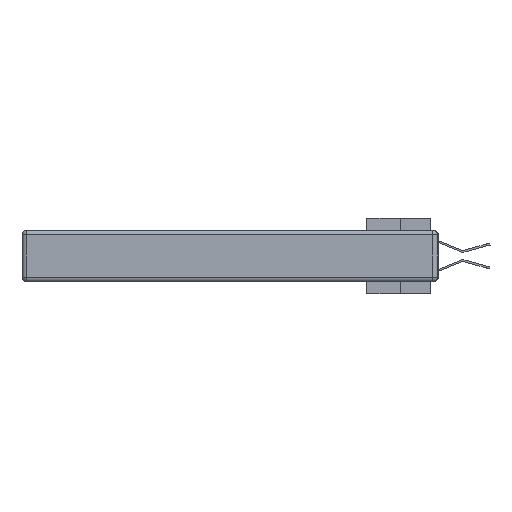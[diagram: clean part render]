
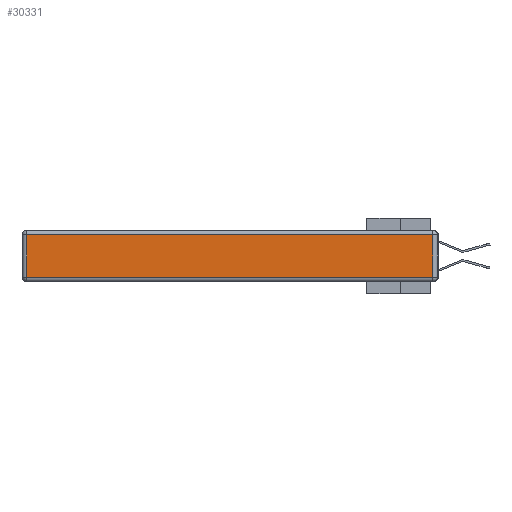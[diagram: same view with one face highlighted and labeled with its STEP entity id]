
A CAD part, left-side view. The second image highlights one B-rep face of the part: STEP entity #30331.
In plain terms, the highlighted planar face has unit normal (-1, 0, 0).
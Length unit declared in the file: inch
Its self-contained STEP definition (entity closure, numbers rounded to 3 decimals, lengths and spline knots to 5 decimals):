
#1260 = VECTOR ( 'NONE', #37777, 39.37008 ) ;
#5420 = CARTESIAN_POINT ( 'NONE',  ( 0., 2.75, -0.03 ) ) ;
#5790 = ORIENTED_EDGE ( 'NONE', *, *, #7274, .T. ) ;
#5884 = DIRECTION ( 'NONE',  ( -1., 0., 0. ) ) ;
#6986 = CARTESIAN_POINT ( 'NONE',  ( 0., 0.03, -0.343 ) ) ;
#7274 = EDGE_CURVE ( 'NONE', #38270, #18598, #39630, .T. ) ;
#7296 = EDGE_CURVE ( 'NONE', #28647, #13485, #34625, .T. ) ;
#8425 = CARTESIAN_POINT ( 'NONE',  ( 0., 0.03, -0.03 ) ) ;
#8587 = VECTOR ( 'NONE', #10253, 39.37008 ) ;
#9181 = ORIENTED_EDGE ( 'NONE', *, *, #15813, .T. ) ;
#10253 = DIRECTION ( 'NONE',  ( 0., 0., 1. ) ) ;
#10560 = CARTESIAN_POINT ( 'NONE',  ( 0., 2.72, -0.03 ) ) ;
#11420 = CARTESIAN_POINT ( 'NONE',  ( 0., 2.72, -0.343 ) ) ;
#11427 = EDGE_LOOP ( 'NONE', ( #5790, #9181, #29926, #25847 ) ) ;
#12086 = DIRECTION ( 'NONE',  ( 0., 1., 0. ) ) ;
#12235 = CARTESIAN_POINT ( 'NONE',  ( 0., 0., -0.313 ) ) ;
#13485 = VERTEX_POINT ( 'NONE', #10560 ) ;
#15813 = EDGE_CURVE ( 'NONE', #18598, #28647, #36400, .T. ) ;
#16239 = LINE ( 'NONE', #11420, #34922 ) ;
#17774 = DIRECTION ( 'NONE',  ( 0., 0., -1. ) ) ;
#18598 = VERTEX_POINT ( 'NONE', #18718 ) ;
#18718 = CARTESIAN_POINT ( 'NONE',  ( 0., 0.03, -0.313 ) ) ;
#21985 = CARTESIAN_POINT ( 'NONE',  ( 0., 0., -0.343 ) ) ;
#23805 = CARTESIAN_POINT ( 'NONE',  ( 0., 2.72, -0.313 ) ) ;
#25847 = ORIENTED_EDGE ( 'NONE', *, *, #31449, .T. ) ;
#28647 = VERTEX_POINT ( 'NONE', #8425 ) ;
#29926 = ORIENTED_EDGE ( 'NONE', *, *, #7296, .T. ) ;
#30135 = AXIS2_PLACEMENT_3D ( 'NONE', #21985, #5884, #31745 ) ;
#30331 = ADVANCED_FACE ( 'NONE', ( #33484 ), #37946, .T. ) ;
#31449 = EDGE_CURVE ( 'NONE', #13485, #38270, #16239, .T. ) ;
#31745 = DIRECTION ( 'NONE',  ( 0., 0., 1. ) ) ;
#32602 = VECTOR ( 'NONE', #12086, 39.37008 ) ;
#33484 = FACE_OUTER_BOUND ( 'NONE', #11427, .T. ) ;
#34625 = LINE ( 'NONE', #5420, #32602 ) ;
#34922 = VECTOR ( 'NONE', #17774, 39.37008 ) ;
#36400 = LINE ( 'NONE', #6986, #8587 ) ;
#37777 = DIRECTION ( 'NONE',  ( 0., -1., 0. ) ) ;
#37946 = PLANE ( 'NONE',  #30135 ) ;
#38270 = VERTEX_POINT ( 'NONE', #23805 ) ;
#39630 = LINE ( 'NONE', #12235, #1260 ) ;
